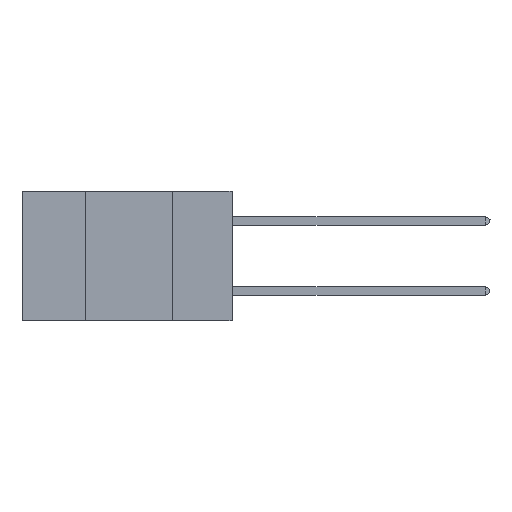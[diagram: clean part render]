
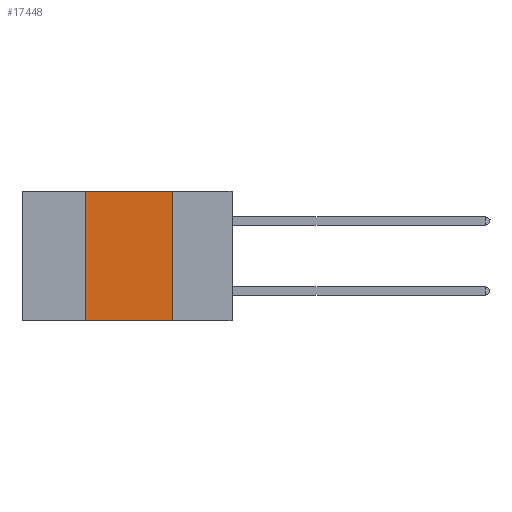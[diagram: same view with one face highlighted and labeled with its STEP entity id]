
A CAD part, left-side view. The second image highlights one B-rep face of the part: STEP entity #17448.
In plain terms, the highlighted planar face has unit normal (-1, 0, 0).
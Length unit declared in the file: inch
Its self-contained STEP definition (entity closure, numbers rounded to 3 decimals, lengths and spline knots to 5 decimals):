
#1596 = ORIENTED_EDGE ( 'NONE', *, *, #35852, .F. ) ;
#4623 = VERTEX_POINT ( 'NONE', #24506 ) ;
#5006 = DIRECTION ( 'NONE',  ( 0., -1., 0. ) ) ;
#5637 = EDGE_CURVE ( 'NONE', #4623, #32187, #22278, .T. ) ;
#5854 = VECTOR ( 'NONE', #5006, 39.37008 ) ;
#6873 = LINE ( 'NONE', #11330, #5854 ) ;
#7164 = ORIENTED_EDGE ( 'NONE', *, *, #34204, .F. ) ;
#7984 = DIRECTION ( 'NONE',  ( 1., 0., 0. ) ) ;
#9421 = CARTESIAN_POINT ( 'NONE',  ( 0., 0.42, 0. ) ) ;
#10170 = ORIENTED_EDGE ( 'NONE', *, *, #39584, .T. ) ;
#10828 = LINE ( 'NONE', #37186, #18929 ) ;
#11330 = CARTESIAN_POINT ( 'NONE',  ( 0., 0.6, -0.37 ) ) ;
#12312 = CARTESIAN_POINT ( 'NONE',  ( 0., 0.17, -0.37 ) ) ;
#12667 = DIRECTION ( 'NONE',  ( 0., 0., 1. ) ) ;
#14669 = CARTESIAN_POINT ( 'NONE',  ( 0., 0.17, 0. ) ) ;
#15352 = VERTEX_POINT ( 'NONE', #39115 ) ;
#17448 = ADVANCED_FACE ( 'NONE', ( #31345 ), #17507, .F. ) ;
#17507 = PLANE ( 'NONE',  #31372 ) ;
#18929 = VECTOR ( 'NONE', #40381, 39.37008 ) ;
#22278 = LINE ( 'NONE', #22650, #29785 ) ;
#22650 = CARTESIAN_POINT ( 'NONE',  ( 0., 0.6, 0. ) ) ;
#24225 = ORIENTED_EDGE ( 'NONE', *, *, #5637, .F. ) ;
#24506 = CARTESIAN_POINT ( 'NONE',  ( 0., 0.42, 0. ) ) ;
#25838 = DIRECTION ( 'NONE',  ( 0., -1., 0. ) ) ;
#26814 = LINE ( 'NONE', #9421, #34327 ) ;
#28049 = VERTEX_POINT ( 'NONE', #12312 ) ;
#29785 = VECTOR ( 'NONE', #25838, 39.37008 ) ;
#30419 = DIRECTION ( 'NONE',  ( 0., 0., -1. ) ) ;
#31345 = FACE_OUTER_BOUND ( 'NONE', #39602, .T. ) ;
#31372 = AXIS2_PLACEMENT_3D ( 'NONE', #36711, #7984, #30419 ) ;
#32187 = VERTEX_POINT ( 'NONE', #14669 ) ;
#34204 = EDGE_CURVE ( 'NONE', #32187, #28049, #10828, .T. ) ;
#34327 = VECTOR ( 'NONE', #12667, 39.37008 ) ;
#35852 = EDGE_CURVE ( 'NONE', #15352, #4623, #26814, .T. ) ;
#36711 = CARTESIAN_POINT ( 'NONE',  ( 0., 0.6, 0. ) ) ;
#37186 = CARTESIAN_POINT ( 'NONE',  ( 0., 0.17, 0. ) ) ;
#39115 = CARTESIAN_POINT ( 'NONE',  ( 0., 0.42, -0.37 ) ) ;
#39584 = EDGE_CURVE ( 'NONE', #15352, #28049, #6873, .T. ) ;
#39602 = EDGE_LOOP ( 'NONE', ( #7164, #24225, #1596, #10170 ) ) ;
#40381 = DIRECTION ( 'NONE',  ( 0., 0., -1. ) ) ;
